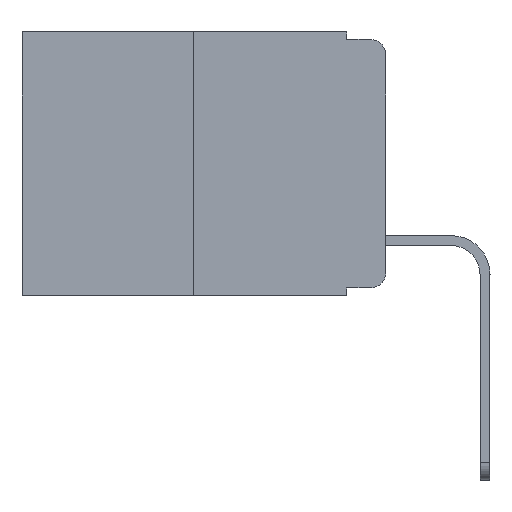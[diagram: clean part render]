
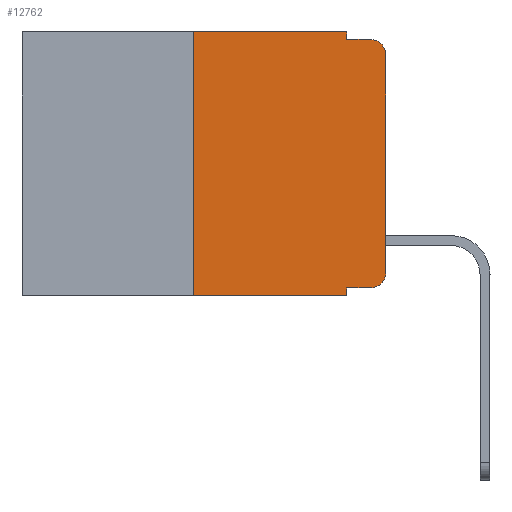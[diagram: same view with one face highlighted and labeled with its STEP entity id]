
A CAD part, left-side view. The second image highlights one B-rep face of the part: STEP entity #12762.
In plain terms, the highlighted planar face has unit normal (-1, 0, 0).
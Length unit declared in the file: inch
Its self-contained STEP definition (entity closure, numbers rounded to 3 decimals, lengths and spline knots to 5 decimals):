
#22 = CARTESIAN_POINT ( 'NONE',  ( 0., 0.25, 0. ) ) ;
#30 = VECTOR ( 'NONE', #14933, 39.37008 ) ;
#120 = EDGE_CURVE ( 'NONE', #10914, #8834, #11621, .T. ) ;
#281 = ORIENTED_EDGE ( 'NONE', *, *, #5692, .T. ) ;
#683 = EDGE_CURVE ( 'NONE', #10329, #8191, #14904, .T. ) ;
#750 = CARTESIAN_POINT ( 'NONE',  ( 0., 0., 0. ) ) ;
#882 = CARTESIAN_POINT ( 'NONE',  ( 0., 0.473, 0. ) ) ;
#910 = CARTESIAN_POINT ( 'NONE',  ( 0., 0.051, -0.343 ) ) ;
#1204 = EDGE_CURVE ( 'NONE', #8834, #10995, #15072, .T. ) ;
#1593 = VERTEX_POINT ( 'NONE', #4120 ) ;
#1960 = CIRCLE ( 'NONE', #6505, 0.02 ) ;
#2180 = AXIS2_PLACEMENT_3D ( 'NONE', #4423, #5608, #10807 ) ;
#2229 = DIRECTION ( 'NONE',  ( 0., -1., 0. ) ) ;
#2640 = DIRECTION ( 'NONE',  ( 0., 0., -1. ) ) ;
#2758 = AXIS2_PLACEMENT_3D ( 'NONE', #15664, #13220, #3197 ) ;
#2814 = VERTEX_POINT ( 'NONE', #9421 ) ;
#3197 = DIRECTION ( 'NONE',  ( 0., 0., -1. ) ) ;
#3715 = VECTOR ( 'NONE', #9461, 39.37008 ) ;
#4120 = CARTESIAN_POINT ( 'NONE',  ( 0., 0.02, -0.333 ) ) ;
#4140 = EDGE_CURVE ( 'NONE', #11326, #15151, #8344, .T. ) ;
#4423 = CARTESIAN_POINT ( 'NONE',  ( 0., 0.473, 0. ) ) ;
#4617 = ORIENTED_EDGE ( 'NONE', *, *, #683, .T. ) ;
#4618 = CARTESIAN_POINT ( 'NONE',  ( 0., 0.02, -0.313 ) ) ;
#5200 = CARTESIAN_POINT ( 'NONE',  ( 0., 0.051, 0. ) ) ;
#5353 = FACE_OUTER_BOUND ( 'NONE', #14615, .T. ) ;
#5608 = DIRECTION ( 'NONE',  ( 1., 0., 0. ) ) ;
#5692 = EDGE_CURVE ( 'NONE', #11326, #1593, #13065, .T. ) ;
#5801 = DIRECTION ( 'NONE',  ( -1., 0., 0. ) ) ;
#5816 = ORIENTED_EDGE ( 'NONE', *, *, #15787, .T. ) ;
#6025 = LINE ( 'NONE', #10001, #30 ) ;
#6080 = VERTEX_POINT ( 'NONE', #15153 ) ;
#6094 = VECTOR ( 'NONE', #6234, 39.37008 ) ;
#6234 = DIRECTION ( 'NONE',  ( 0., 0., 1. ) ) ;
#6254 = CARTESIAN_POINT ( 'NONE',  ( 0., 0., -0.03 ) ) ;
#6505 = AXIS2_PLACEMENT_3D ( 'NONE', #4618, #5801, #7071 ) ;
#6799 = ORIENTED_EDGE ( 'NONE', *, *, #4140, .F. ) ;
#7071 = DIRECTION ( 'NONE',  ( 0., 0., -1. ) ) ;
#7215 = CARTESIAN_POINT ( 'NONE',  ( 0., 0.051, -0.333 ) ) ;
#7257 = ORIENTED_EDGE ( 'NONE', *, *, #10315, .T. ) ;
#7590 = VECTOR ( 'NONE', #2229, 39.37008 ) ;
#7850 = CARTESIAN_POINT ( 'NONE',  ( 0., 0.051, -0.01 ) ) ;
#7899 = VECTOR ( 'NONE', #13994, 39.37008 ) ;
#8191 = VERTEX_POINT ( 'NONE', #6254 ) ;
#8290 = CARTESIAN_POINT ( 'NONE',  ( 0., 0.051, -0.01 ) ) ;
#8308 = CARTESIAN_POINT ( 'NONE',  ( 0., 0., -0.313 ) ) ;
#8344 = LINE ( 'NONE', #13646, #13934 ) ;
#8834 = VERTEX_POINT ( 'NONE', #5200 ) ;
#9152 = EDGE_CURVE ( 'NONE', #8191, #6080, #12030, .T. ) ;
#9389 = LINE ( 'NONE', #22, #6094 ) ;
#9421 = CARTESIAN_POINT ( 'NONE',  ( 0., 0.25, -0.343 ) ) ;
#9461 = DIRECTION ( 'NONE',  ( 0., 0., 1. ) ) ;
#10001 = CARTESIAN_POINT ( 'NONE',  ( 0., 0.473, -0.343 ) ) ;
#10150 = ORIENTED_EDGE ( 'NONE', *, *, #120, .F. ) ;
#10207 = ORIENTED_EDGE ( 'NONE', *, *, #14045, .F. ) ;
#10315 = EDGE_CURVE ( 'NONE', #1593, #10329, #1960, .T. ) ;
#10329 = VERTEX_POINT ( 'NONE', #8308 ) ;
#10807 = DIRECTION ( 'NONE',  ( 0., 0., -1. ) ) ;
#10914 = VERTEX_POINT ( 'NONE', #15997 ) ;
#10995 = VERTEX_POINT ( 'NONE', #8290 ) ;
#11169 = LINE ( 'NONE', #7850, #7899 ) ;
#11217 = VECTOR ( 'NONE', #2640, 39.37008 ) ;
#11326 = VERTEX_POINT ( 'NONE', #13038 ) ;
#11621 = LINE ( 'NONE', #882, #7590 ) ;
#12030 = CIRCLE ( 'NONE', #2758, 0.02 ) ;
#12062 = ORIENTED_EDGE ( 'NONE', *, *, #1204, .F. ) ;
#12287 = ORIENTED_EDGE ( 'NONE', *, *, #12583, .F. ) ;
#12583 = EDGE_CURVE ( 'NONE', #10995, #6080, #11169, .T. ) ;
#12762 = ADVANCED_FACE ( 'NONE', ( #5353 ), #13155, .F. ) ;
#13038 = CARTESIAN_POINT ( 'NONE',  ( 0., 0.051, -0.333 ) ) ;
#13065 = LINE ( 'NONE', #7215, #14258 ) ;
#13155 = PLANE ( 'NONE',  #2180 ) ;
#13220 = DIRECTION ( 'NONE',  ( -1., 0., 0. ) ) ;
#13450 = ORIENTED_EDGE ( 'NONE', *, *, #9152, .T. ) ;
#13646 = CARTESIAN_POINT ( 'NONE',  ( 0., 0.051, 0. ) ) ;
#13934 = VECTOR ( 'NONE', #14750, 39.37008 ) ;
#13994 = DIRECTION ( 'NONE',  ( 0., -1., 0. ) ) ;
#14045 = EDGE_CURVE ( 'NONE', #2814, #10914, #9389, .T. ) ;
#14258 = VECTOR ( 'NONE', #14428, 39.37008 ) ;
#14428 = DIRECTION ( 'NONE',  ( 0., -1., 0. ) ) ;
#14615 = EDGE_LOOP ( 'NONE', ( #4617, #13450, #12287, #12062, #10150, #10207, #5816, #6799, #281, #7257 ) ) ;
#14750 = DIRECTION ( 'NONE',  ( 0., 0., -1. ) ) ;
#14904 = LINE ( 'NONE', #750, #3715 ) ;
#14933 = DIRECTION ( 'NONE',  ( 0., -1., 0. ) ) ;
#15072 = LINE ( 'NONE', #15155, #11217 ) ;
#15151 = VERTEX_POINT ( 'NONE', #910 ) ;
#15153 = CARTESIAN_POINT ( 'NONE',  ( 0., 0.02, -0.01 ) ) ;
#15155 = CARTESIAN_POINT ( 'NONE',  ( 0., 0.051, 0. ) ) ;
#15664 = CARTESIAN_POINT ( 'NONE',  ( 0., 0.02, -0.03 ) ) ;
#15787 = EDGE_CURVE ( 'NONE', #2814, #15151, #6025, .T. ) ;
#15997 = CARTESIAN_POINT ( 'NONE',  ( 0., 0.25, 0. ) ) ;
